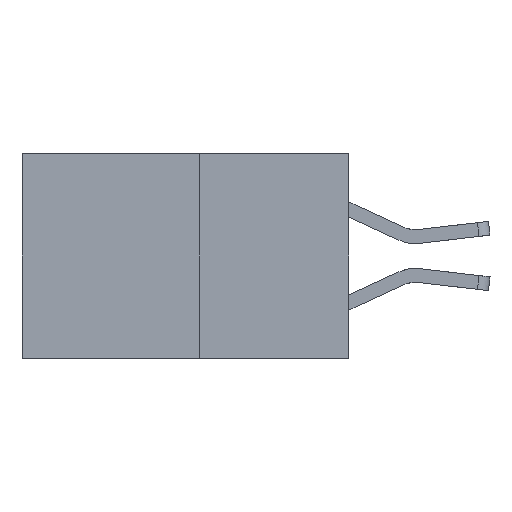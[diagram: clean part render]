
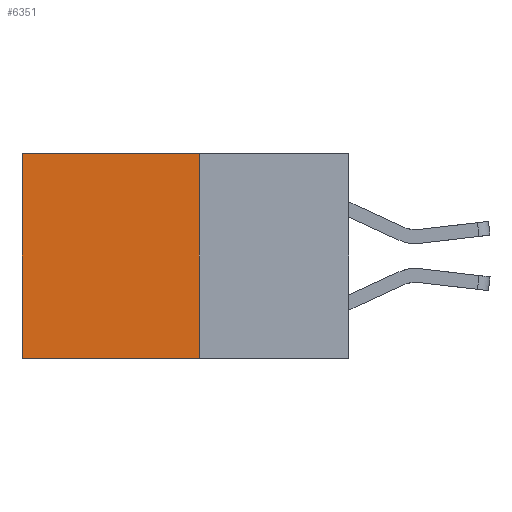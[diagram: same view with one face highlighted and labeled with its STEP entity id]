
A CAD part, left-side view. The second image highlights one B-rep face of the part: STEP entity #6351.
In plain terms, the highlighted planar face has unit normal (-1, 0, 0).
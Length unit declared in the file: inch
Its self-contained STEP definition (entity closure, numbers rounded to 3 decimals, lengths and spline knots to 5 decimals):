
#377 = CARTESIAN_POINT ( 'NONE',  ( 0.277, 0.59, 0. ) ) ;
#832 = EDGE_CURVE ( 'NONE', #5021, #7154, #6912, .T. ) ;
#1325 = DIRECTION ( 'NONE',  ( 0., 1., 0. ) ) ;
#1560 = DIRECTION ( 'NONE',  ( 1., 0., 0. ) ) ;
#1569 = FACE_OUTER_BOUND ( 'NONE', #2783, .T. ) ;
#1825 = LINE ( 'NONE', #7354, #7360 ) ;
#2783 = EDGE_LOOP ( 'NONE', ( #4347, #4567, #4636, #4860 ) ) ;
#3365 = VERTEX_POINT ( 'NONE', #377 ) ;
#3627 = DIRECTION ( 'NONE',  ( 0., 0., -1. ) ) ;
#3861 = CARTESIAN_POINT ( 'NONE',  ( 0.277, 0.27, -0.37 ) ) ;
#4225 = CARTESIAN_POINT ( 'NONE',  ( 0.277, 0.27, 0. ) ) ;
#4347 = ORIENTED_EDGE ( 'NONE', *, *, #4975, .T. ) ;
#4500 = DIRECTION ( 'NONE',  ( 0., 0., -1. ) ) ;
#4567 = ORIENTED_EDGE ( 'NONE', *, *, #832, .F. ) ;
#4636 = ORIENTED_EDGE ( 'NONE', *, *, #6240, .F. ) ;
#4753 = EDGE_CURVE ( 'NONE', #6534, #3365, #5769, .T. ) ;
#4860 = ORIENTED_EDGE ( 'NONE', *, *, #4753, .T. ) ;
#4863 = VECTOR ( 'NONE', #3627, 39.37008 ) ;
#4975 = EDGE_CURVE ( 'NONE', #3365, #7154, #1825, .T. ) ;
#5021 = VERTEX_POINT ( 'NONE', #3861 ) ;
#5752 = CARTESIAN_POINT ( 'NONE',  ( 0.277, 0.27, -0.37 ) ) ;
#5769 = LINE ( 'NONE', #4225, #7477 ) ;
#5864 = AXIS2_PLACEMENT_3D ( 'NONE', #5881, #1560, #6626 ) ;
#5881 = CARTESIAN_POINT ( 'NONE',  ( 0.277, 0.27, -0.37 ) ) ;
#6061 = CARTESIAN_POINT ( 'NONE',  ( 0.277, 0.27, 0. ) ) ;
#6240 = EDGE_CURVE ( 'NONE', #6534, #5021, #8427, .T. ) ;
#6351 = ADVANCED_FACE ( 'NONE', ( #1569 ), #8026, .F. ) ;
#6534 = VERTEX_POINT ( 'NONE', #6061 ) ;
#6626 = DIRECTION ( 'NONE',  ( 0., 0., -1. ) ) ;
#6763 = CARTESIAN_POINT ( 'NONE',  ( 0.277, 0.59, -0.37 ) ) ;
#6912 = LINE ( 'NONE', #5752, #8580 ) ;
#7154 = VERTEX_POINT ( 'NONE', #6763 ) ;
#7354 = CARTESIAN_POINT ( 'NONE',  ( 0.277, 0.59, -0.37 ) ) ;
#7360 = VECTOR ( 'NONE', #4500, 39.37008 ) ;
#7386 = DIRECTION ( 'NONE',  ( 0., 1., 0. ) ) ;
#7477 = VECTOR ( 'NONE', #1325, 39.37008 ) ;
#7903 = CARTESIAN_POINT ( 'NONE',  ( 0.277, 0.27, -0.37 ) ) ;
#8026 = PLANE ( 'NONE',  #5864 ) ;
#8427 = LINE ( 'NONE', #7903, #4863 ) ;
#8580 = VECTOR ( 'NONE', #7386, 39.37008 ) ;
